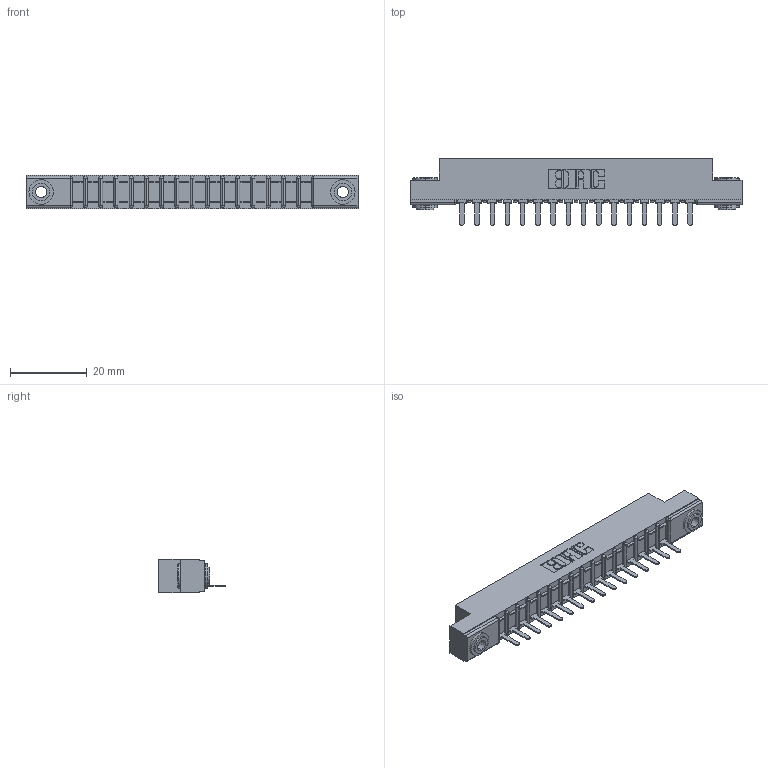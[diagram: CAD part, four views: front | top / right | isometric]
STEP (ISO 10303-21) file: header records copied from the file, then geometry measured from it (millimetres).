
FILE_DESCRIPTION (( 'STEP AP203' ), '1' );
FILE_NAME ('357-016-521-103.STEP', '2019-09-16T20:37:01', ( '' ), ( '' ), 'SwSTEP 2.0', 'SolidWorks 2016', '' );
FILE_SCHEMA (( 'CONFIG_CONTROL_DESIGN' ));
Length unit declared in the file: inch
Products named in the file (4): 345-250-002_345-250-002-102; 357-016-521-103; 307-290-002_521; 307 Part_.156 Dia Mounting Holes
Assembly tree (19 placements, depth 2):
  357-016-521-103
    307 Part_.156 Dia Mounting Holes
    307-290-002_521  x16
    345-250-002_345-250-002-102  x2
Bounding box: 86.41 x 17.42 x 8.71 mm (x, y, z)
Volume: 5703.8 mm3; surface area: 10294.1 mm2
Topology: 19 solids, 19 shells, 1371 faces, 4147 edges, 2714 vertices
Faces by surface type: plane 814, cylinder 515, sphere 34, cone 8
Entity records: 18705 total; most frequent: CARTESIAN_POINT 3129, ORIENTED_EDGE 3110, DIRECTION 3067, EDGE_CURVE 1555, VECTOR 1171, LINE 1171, VERTEX_POINT 1010, AXIS2_PLACEMENT_3D 948
